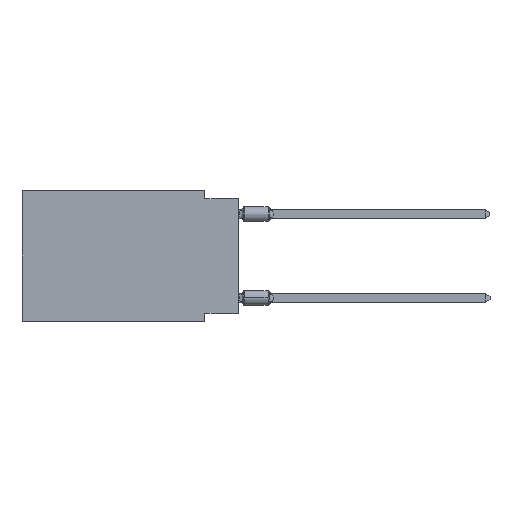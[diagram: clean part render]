
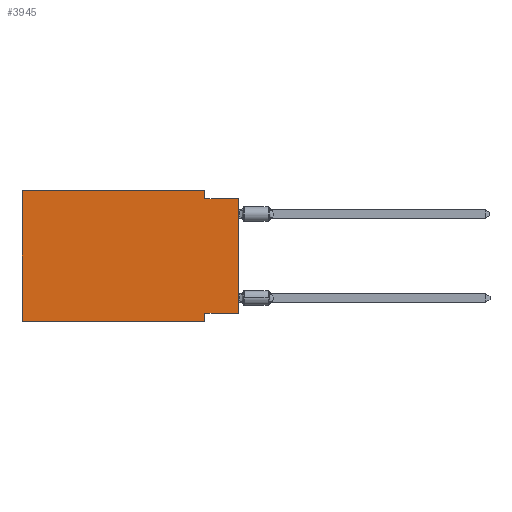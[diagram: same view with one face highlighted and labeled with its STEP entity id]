
A CAD part, left-side view. The second image highlights one B-rep face of the part: STEP entity #3945.
In plain terms, the highlighted planar face has unit normal (-1, 0, 0).
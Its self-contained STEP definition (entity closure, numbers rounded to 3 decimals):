
#329 = CARTESIAN_POINT ( 'NONE',  ( 0., 2.54, -9.906 ) ) ;
#1544 = ORIENTED_EDGE ( 'NONE', *, *, #8596, .F. ) ;
#2041 = CARTESIAN_POINT ( 'NONE',  ( 0., 0., -9.271 ) ) ;
#2095 = EDGE_CURVE ( 'NONE', #6784, #6649, #21363, .T. ) ;
#2245 = CARTESIAN_POINT ( 'NONE',  ( 0., 16.383, -9.906 ) ) ;
#2671 = VERTEX_POINT ( 'NONE', #10177 ) ;
#2994 = DIRECTION ( 'NONE',  ( 0., -1., 0. ) ) ;
#3163 = EDGE_CURVE ( 'NONE', #16487, #20582, #23465, .T. ) ;
#3945 = ADVANCED_FACE ( 'NONE', ( #10095 ), #8230, .F. ) ;
#4119 = CARTESIAN_POINT ( 'NONE',  ( 0., 16.383, 0. ) ) ;
#4140 = VECTOR ( 'NONE', #6903, 1000. ) ;
#4578 = EDGE_CURVE ( 'NONE', #12349, #20582, #12295, .T. ) ;
#4961 = CARTESIAN_POINT ( 'NONE',  ( 0., 16.383, 0. ) ) ;
#5322 = ORIENTED_EDGE ( 'NONE', *, *, #6724, .F. ) ;
#5481 = CARTESIAN_POINT ( 'NONE',  ( 0., 0., -9.271 ) ) ;
#5726 = ORIENTED_EDGE ( 'NONE', *, *, #2095, .F. ) ;
#6649 = VERTEX_POINT ( 'NONE', #12716 ) ;
#6724 = EDGE_CURVE ( 'NONE', #16487, #6784, #14449, .T. ) ;
#6733 = CARTESIAN_POINT ( 'NONE',  ( 0., 0., -0.635 ) ) ;
#6784 = VERTEX_POINT ( 'NONE', #13581 ) ;
#6889 = ORIENTED_EDGE ( 'NONE', *, *, #19521, .F. ) ;
#6903 = DIRECTION ( 'NONE',  ( 0., -1., 0. ) ) ;
#7917 = EDGE_CURVE ( 'NONE', #16723, #12349, #10991, .T. ) ;
#8230 = PLANE ( 'NONE',  #11553 ) ;
#8596 = EDGE_CURVE ( 'NONE', #2671, #16723, #17918, .T. ) ;
#9834 = VERTEX_POINT ( 'NONE', #2245 ) ;
#10095 = FACE_OUTER_BOUND ( 'NONE', #14824, .T. ) ;
#10177 = CARTESIAN_POINT ( 'NONE',  ( 0., 16.383, 0. ) ) ;
#10509 = CARTESIAN_POINT ( 'NONE',  ( 0., 0., 0. ) ) ;
#10629 = DIRECTION ( 'NONE',  ( 0., 0., -1. ) ) ;
#10693 = CARTESIAN_POINT ( 'NONE',  ( 0., 2.54, 0. ) ) ;
#10991 = LINE ( 'NONE', #14557, #12342 ) ;
#11553 = AXIS2_PLACEMENT_3D ( 'NONE', #15838, #21457, #11937 ) ;
#11839 = ORIENTED_EDGE ( 'NONE', *, *, #14035, .T. ) ;
#11937 = DIRECTION ( 'NONE',  ( 0., 0., -1. ) ) ;
#12295 = LINE ( 'NONE', #19758, #13920 ) ;
#12342 = VECTOR ( 'NONE', #10629, 1000. ) ;
#12349 = VERTEX_POINT ( 'NONE', #16852 ) ;
#12716 = CARTESIAN_POINT ( 'NONE',  ( 0., 2.54, -9.906 ) ) ;
#12728 = VECTOR ( 'NONE', #23428, 1000. ) ;
#13581 = CARTESIAN_POINT ( 'NONE',  ( 0., 2.54, -9.271 ) ) ;
#13920 = VECTOR ( 'NONE', #2994, 1000. ) ;
#14035 = EDGE_CURVE ( 'NONE', #9834, #6649, #15973, .T. ) ;
#14188 = DIRECTION ( 'NONE',  ( 0., 0., 1. ) ) ;
#14363 = ORIENTED_EDGE ( 'NONE', *, *, #4578, .F. ) ;
#14449 = LINE ( 'NONE', #5481, #15789 ) ;
#14557 = CARTESIAN_POINT ( 'NONE',  ( 0., 2.54, 0. ) ) ;
#14824 = EDGE_LOOP ( 'NONE', ( #16179, #14363, #17122, #1544, #6889, #11839, #5726, #5322 ) ) ;
#15512 = LINE ( 'NONE', #4119, #20849 ) ;
#15789 = VECTOR ( 'NONE', #18219, 1000. ) ;
#15838 = CARTESIAN_POINT ( 'NONE',  ( 0., 16.383, 0. ) ) ;
#15973 = LINE ( 'NONE', #22719, #12728 ) ;
#16179 = ORIENTED_EDGE ( 'NONE', *, *, #3163, .T. ) ;
#16487 = VERTEX_POINT ( 'NONE', #2041 ) ;
#16723 = VERTEX_POINT ( 'NONE', #10693 ) ;
#16852 = CARTESIAN_POINT ( 'NONE',  ( 0., 2.54, -0.635 ) ) ;
#17122 = ORIENTED_EDGE ( 'NONE', *, *, #7917, .F. ) ;
#17207 = DIRECTION ( 'NONE',  ( 0., 0., 1. ) ) ;
#17918 = LINE ( 'NONE', #4961, #4140 ) ;
#18155 = VECTOR ( 'NONE', #14188, 1000. ) ;
#18219 = DIRECTION ( 'NONE',  ( 0., 1., 0. ) ) ;
#19521 = EDGE_CURVE ( 'NONE', #9834, #2671, #15512, .T. ) ;
#19758 = CARTESIAN_POINT ( 'NONE',  ( 0., 0., -0.635 ) ) ;
#20582 = VERTEX_POINT ( 'NONE', #6733 ) ;
#20849 = VECTOR ( 'NONE', #17207, 1000. ) ;
#21363 = LINE ( 'NONE', #329, #22625 ) ;
#21457 = DIRECTION ( 'NONE',  ( 1., 0., 0. ) ) ;
#22625 = VECTOR ( 'NONE', #22829, 1000. ) ;
#22719 = CARTESIAN_POINT ( 'NONE',  ( 0., 16.383, -9.906 ) ) ;
#22829 = DIRECTION ( 'NONE',  ( 0., 0., -1. ) ) ;
#23428 = DIRECTION ( 'NONE',  ( 0., -1., 0. ) ) ;
#23465 = LINE ( 'NONE', #10509, #18155 ) ;
